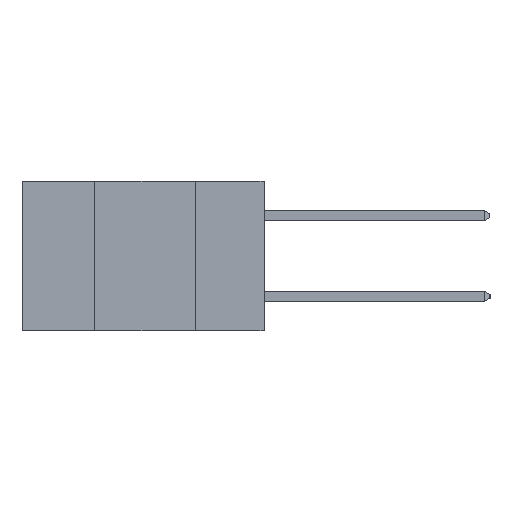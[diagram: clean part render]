
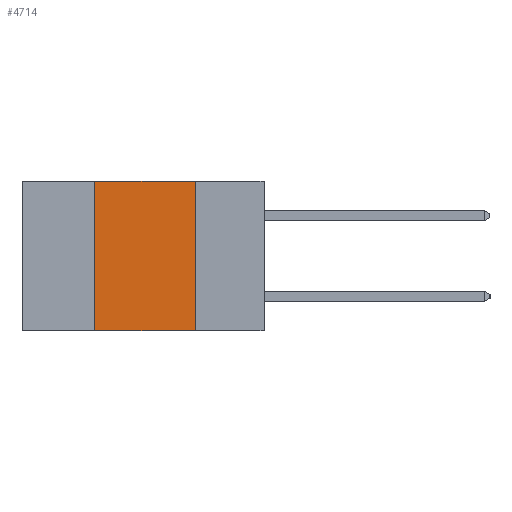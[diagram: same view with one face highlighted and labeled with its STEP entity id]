
A CAD part, left-side view. The second image highlights one B-rep face of the part: STEP entity #4714.
In plain terms, the highlighted planar face has unit normal (-1, 0, 0).
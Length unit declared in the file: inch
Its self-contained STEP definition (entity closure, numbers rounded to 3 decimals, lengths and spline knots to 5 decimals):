
#193 = LINE ( 'NONE', #4097, #11228 ) ;
#329 = VERTEX_POINT ( 'NONE', #8844 ) ;
#650 = VERTEX_POINT ( 'NONE', #3246 ) ;
#807 = EDGE_LOOP ( 'NONE', ( #10620, #13257, #8309, #10948 ) ) ;
#992 = DIRECTION ( 'NONE',  ( 0., 0., -1. ) ) ;
#1035 = DIRECTION ( 'NONE',  ( 1., 0., 0. ) ) ;
#1095 = PLANE ( 'NONE',  #12613 ) ;
#1781 = CARTESIAN_POINT ( 'NONE',  ( 0., 0.6, 0. ) ) ;
#1998 = LINE ( 'NONE', #10557, #7041 ) ;
#2584 = CARTESIAN_POINT ( 'NONE',  ( 0., 0.17, -0.37 ) ) ;
#3246 = CARTESIAN_POINT ( 'NONE',  ( 0., 0.42, -0.37 ) ) ;
#3670 = FACE_OUTER_BOUND ( 'NONE', #807, .T. ) ;
#4097 = CARTESIAN_POINT ( 'NONE',  ( 0., 0.17, -0.37 ) ) ;
#4329 = CARTESIAN_POINT ( 'NONE',  ( 0., 0.6, 0. ) ) ;
#4376 = DIRECTION ( 'NONE',  ( 0., 0., 1. ) ) ;
#4471 = DIRECTION ( 'NONE',  ( 0., -1., 0. ) ) ;
#4714 = ADVANCED_FACE ( 'NONE', ( #3670 ), #1095, .F. ) ;
#4874 = VECTOR ( 'NONE', #4376, 39.37008 ) ;
#4978 = VERTEX_POINT ( 'NONE', #10926 ) ;
#6535 = CARTESIAN_POINT ( 'NONE',  ( 0., 0.42, -0.37 ) ) ;
#7041 = VECTOR ( 'NONE', #4471, 39.37008 ) ;
#7960 = LINE ( 'NONE', #4329, #10577 ) ;
#8196 = EDGE_CURVE ( 'NONE', #4978, #9901, #193, .T. ) ;
#8213 = EDGE_CURVE ( 'NONE', #329, #4978, #7960, .T. ) ;
#8234 = EDGE_CURVE ( 'NONE', #650, #329, #10256, .T. ) ;
#8272 = EDGE_CURVE ( 'NONE', #650, #9901, #1998, .T. ) ;
#8309 = ORIENTED_EDGE ( 'NONE', *, *, #8234, .F. ) ;
#8844 = CARTESIAN_POINT ( 'NONE',  ( 0., 0.42, 0. ) ) ;
#9901 = VERTEX_POINT ( 'NONE', #2584 ) ;
#10256 = LINE ( 'NONE', #6535, #4874 ) ;
#10557 = CARTESIAN_POINT ( 'NONE',  ( 0., 0.6, -0.37 ) ) ;
#10577 = VECTOR ( 'NONE', #11493, 39.37008 ) ;
#10620 = ORIENTED_EDGE ( 'NONE', *, *, #8196, .F. ) ;
#10926 = CARTESIAN_POINT ( 'NONE',  ( 0., 0.17, 0. ) ) ;
#10948 = ORIENTED_EDGE ( 'NONE', *, *, #8272, .T. ) ;
#11228 = VECTOR ( 'NONE', #11243, 39.37008 ) ;
#11243 = DIRECTION ( 'NONE',  ( 0., 0., -1. ) ) ;
#11493 = DIRECTION ( 'NONE',  ( 0., -1., 0. ) ) ;
#12613 = AXIS2_PLACEMENT_3D ( 'NONE', #1781, #1035, #992 ) ;
#13257 = ORIENTED_EDGE ( 'NONE', *, *, #8213, .F. ) ;
